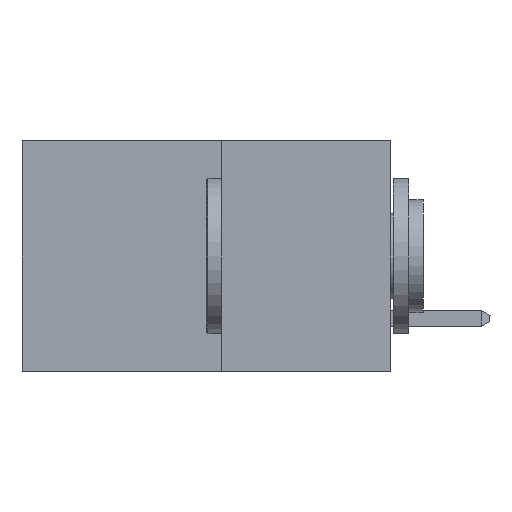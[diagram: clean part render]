
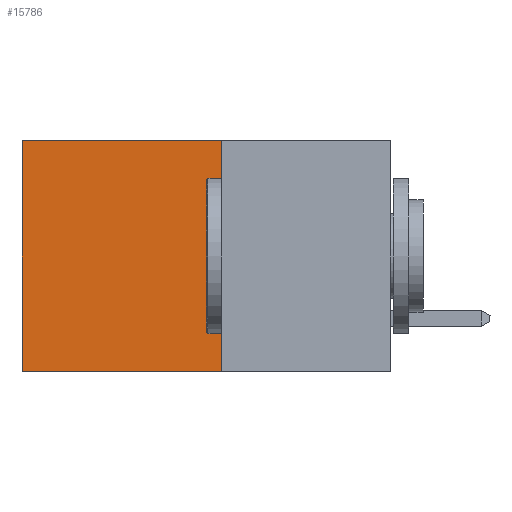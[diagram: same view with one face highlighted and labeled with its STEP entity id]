
A CAD part, left-side view. The second image highlights one B-rep face of the part: STEP entity #15786.
In plain terms, the highlighted planar face has unit normal (-1, 0, 0).
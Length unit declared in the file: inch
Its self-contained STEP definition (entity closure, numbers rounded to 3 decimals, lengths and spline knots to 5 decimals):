
#873 = DIRECTION ( 'NONE',  ( 0., 0., -1. ) ) ;
#2825 = DIRECTION ( 'NONE',  ( 0., 0., -1. ) ) ;
#2827 = VECTOR ( 'NONE', #5706, 39.37008 ) ;
#3337 = CARTESIAN_POINT ( 'NONE',  ( 0.277, 0.59, -0.37 ) ) ;
#3949 = VERTEX_POINT ( 'NONE', #17707 ) ;
#5706 = DIRECTION ( 'NONE',  ( 0., 1., 0. ) ) ;
#6269 = EDGE_LOOP ( 'NONE', ( #7142, #8214, #25999, #21216 ) ) ;
#6907 = CARTESIAN_POINT ( 'NONE',  ( 0.277, 0.59, 0. ) ) ;
#7072 = AXIS2_PLACEMENT_3D ( 'NONE', #13323, #15402, #2825 ) ;
#7142 = ORIENTED_EDGE ( 'NONE', *, *, #25207, .T. ) ;
#7681 = LINE ( 'NONE', #25191, #18141 ) ;
#8214 = ORIENTED_EDGE ( 'NONE', *, *, #23174, .F. ) ;
#8479 = LINE ( 'NONE', #24414, #2827 ) ;
#8782 = VERTEX_POINT ( 'NONE', #6907 ) ;
#9667 = VERTEX_POINT ( 'NONE', #18188 ) ;
#11592 = LINE ( 'NONE', #26004, #22650 ) ;
#13283 = VECTOR ( 'NONE', #18775, 39.37008 ) ;
#13323 = CARTESIAN_POINT ( 'NONE',  ( 0.277, 0.27, -0.37 ) ) ;
#14809 = VERTEX_POINT ( 'NONE', #3337 ) ;
#14816 = DIRECTION ( 'NONE',  ( 0., 0., -1. ) ) ;
#15402 = DIRECTION ( 'NONE',  ( 1., 0., 0. ) ) ;
#15786 = ADVANCED_FACE ( 'NONE', ( #26062 ), #25796, .F. ) ;
#17707 = CARTESIAN_POINT ( 'NONE',  ( 0.277, 0.27, -0.37 ) ) ;
#18141 = VECTOR ( 'NONE', #14816, 39.37008 ) ;
#18188 = CARTESIAN_POINT ( 'NONE',  ( 0.277, 0.27, 0. ) ) ;
#18775 = DIRECTION ( 'NONE',  ( 0., 1., 0. ) ) ;
#19012 = EDGE_CURVE ( 'NONE', #9667, #8782, #20108, .T. ) ;
#20108 = LINE ( 'NONE', #27064, #13283 ) ;
#21216 = ORIENTED_EDGE ( 'NONE', *, *, #19012, .T. ) ;
#22650 = VECTOR ( 'NONE', #873, 39.37008 ) ;
#23174 = EDGE_CURVE ( 'NONE', #3949, #14809, #8479, .T. ) ;
#24414 = CARTESIAN_POINT ( 'NONE',  ( 0.277, 0.27, -0.37 ) ) ;
#25191 = CARTESIAN_POINT ( 'NONE',  ( 0.277, 0.59, -0.37 ) ) ;
#25207 = EDGE_CURVE ( 'NONE', #8782, #14809, #7681, .T. ) ;
#25452 = EDGE_CURVE ( 'NONE', #9667, #3949, #11592, .T. ) ;
#25796 = PLANE ( 'NONE',  #7072 ) ;
#25999 = ORIENTED_EDGE ( 'NONE', *, *, #25452, .F. ) ;
#26004 = CARTESIAN_POINT ( 'NONE',  ( 0.277, 0.27, -0.37 ) ) ;
#26062 = FACE_OUTER_BOUND ( 'NONE', #6269, .T. ) ;
#27064 = CARTESIAN_POINT ( 'NONE',  ( 0.277, 0.27, 0. ) ) ;
